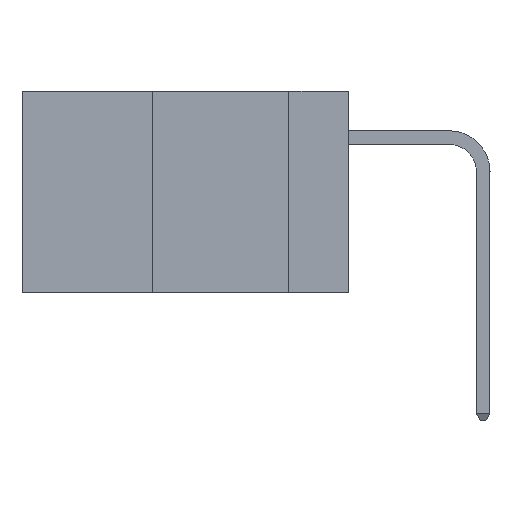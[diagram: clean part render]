
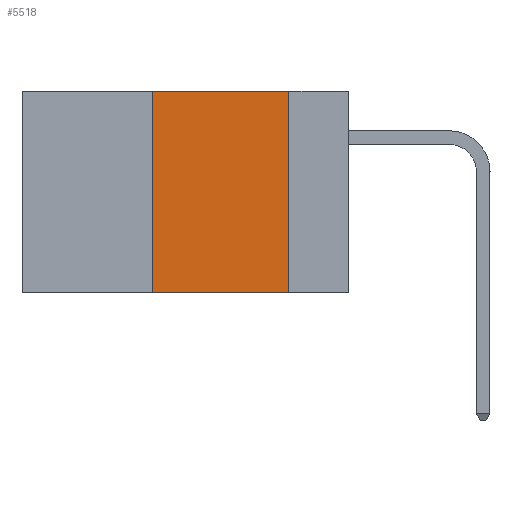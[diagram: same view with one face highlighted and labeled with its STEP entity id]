
A CAD part, left-side view. The second image highlights one B-rep face of the part: STEP entity #5518.
In plain terms, the highlighted planar face has unit normal (-1, 0, 0).
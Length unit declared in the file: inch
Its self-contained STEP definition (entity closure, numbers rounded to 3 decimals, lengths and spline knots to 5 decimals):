
#48 = DIRECTION ( 'NONE',  ( 0., 0., 1. ) ) ;
#1091 = DIRECTION ( 'NONE',  ( 0., 0., -1. ) ) ;
#1438 = CARTESIAN_POINT ( 'NONE',  ( 0., 0.6, 0. ) ) ;
#1752 = VERTEX_POINT ( 'NONE', #15918 ) ;
#2756 = VERTEX_POINT ( 'NONE', #3018 ) ;
#2956 = VECTOR ( 'NONE', #7566, 39.37008 ) ;
#3018 = CARTESIAN_POINT ( 'NONE',  ( 0., 0.11, -0.37 ) ) ;
#3413 = CARTESIAN_POINT ( 'NONE',  ( 0., 0.11, 0. ) ) ;
#3451 = EDGE_CURVE ( 'NONE', #17977, #1752, #17552, .T. ) ;
#4955 = CARTESIAN_POINT ( 'NONE',  ( 0., 0.36, -0.37 ) ) ;
#5239 = VERTEX_POINT ( 'NONE', #11805 ) ;
#5307 = AXIS2_PLACEMENT_3D ( 'NONE', #29335, #15251, #1091 ) ;
#5518 = ADVANCED_FACE ( 'NONE', ( #14536 ), #12859, .F. ) ;
#6188 = DIRECTION ( 'NONE',  ( 0., -1., 0. ) ) ;
#6935 = LINE ( 'NONE', #3413, #30510 ) ;
#7566 = DIRECTION ( 'NONE',  ( 0., -1., 0. ) ) ;
#9174 = LINE ( 'NONE', #14583, #2956 ) ;
#11269 = VECTOR ( 'NONE', #48, 39.37008 ) ;
#11805 = CARTESIAN_POINT ( 'NONE',  ( 0., 0.11, 0. ) ) ;
#12859 = PLANE ( 'NONE',  #5307 ) ;
#14536 = FACE_OUTER_BOUND ( 'NONE', #25864, .T. ) ;
#14583 = CARTESIAN_POINT ( 'NONE',  ( 0., 0.6, -0.37 ) ) ;
#15251 = DIRECTION ( 'NONE',  ( 1., 0., 0. ) ) ;
#15918 = CARTESIAN_POINT ( 'NONE',  ( 0., 0.36, 0. ) ) ;
#16840 = ORIENTED_EDGE ( 'NONE', *, *, #3451, .F. ) ;
#17552 = LINE ( 'NONE', #30446, #11269 ) ;
#17977 = VERTEX_POINT ( 'NONE', #4955 ) ;
#18105 = ORIENTED_EDGE ( 'NONE', *, *, #21480, .F. ) ;
#18782 = EDGE_CURVE ( 'NONE', #5239, #2756, #6935, .T. ) ;
#19728 = DIRECTION ( 'NONE',  ( 0., 0., -1. ) ) ;
#20853 = VECTOR ( 'NONE', #6188, 39.37008 ) ;
#21480 = EDGE_CURVE ( 'NONE', #1752, #5239, #27184, .T. ) ;
#23056 = ORIENTED_EDGE ( 'NONE', *, *, #26134, .T. ) ;
#25864 = EDGE_LOOP ( 'NONE', ( #26729, #18105, #16840, #23056 ) ) ;
#26134 = EDGE_CURVE ( 'NONE', #17977, #2756, #9174, .T. ) ;
#26729 = ORIENTED_EDGE ( 'NONE', *, *, #18782, .F. ) ;
#27184 = LINE ( 'NONE', #1438, #20853 ) ;
#29335 = CARTESIAN_POINT ( 'NONE',  ( 0., 0.6, 0. ) ) ;
#30446 = CARTESIAN_POINT ( 'NONE',  ( 0., 0.36, 0. ) ) ;
#30510 = VECTOR ( 'NONE', #19728, 39.37008 ) ;
